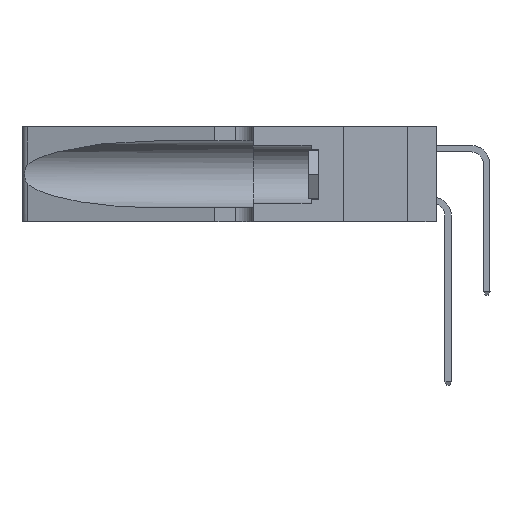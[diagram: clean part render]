
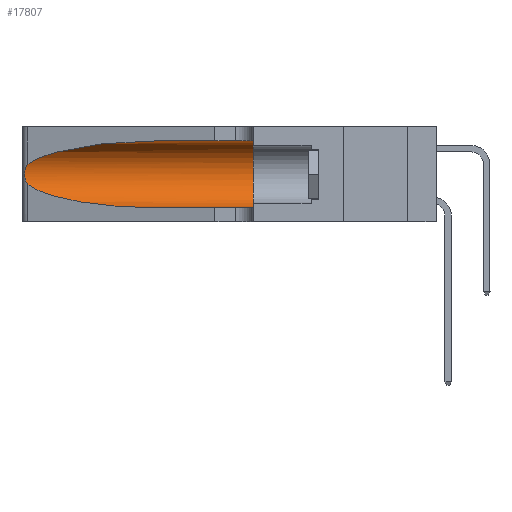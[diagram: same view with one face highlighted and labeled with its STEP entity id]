
A CAD part, left-side view. The second image highlights one B-rep face of the part: STEP entity #17807.
In plain terms, the highlighted cylindrical face has radius 3.308 mm (diameter 6.617 mm), a partial arc.
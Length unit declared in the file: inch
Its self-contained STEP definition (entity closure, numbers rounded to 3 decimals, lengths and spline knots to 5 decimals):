
#35 = CARTESIAN_POINT ( 'NONE',  ( 0.18966, 0.96281, 0.05475 ) ) ;
#333 = VERTEX_POINT ( 'NONE', #11581 ) ;
#340 = EDGE_CURVE ( 'NONE', #333, #13767, #14621, .T. ) ;
#461 = ORIENTED_EDGE ( 'NONE', *, *, #8582, .T. ) ;
#627 = CARTESIAN_POINT ( 'NONE',  ( 0.25487, 1.22718, 0.14631 ) ) ;
#986 = DIRECTION ( 'NONE',  ( 0., -1., 0. ) ) ;
#1318 = CARTESIAN_POINT ( 'NONE',  ( 0.25555, 1.22994, 0.2215 ) ) ;
#1397 = CARTESIAN_POINT ( 'NONE',  ( 0.25639, 1.23186, 0.15144 ) ) ;
#1609 =( BOUNDED_CURVE ( )  B_SPLINE_CURVE ( 3, ( #13322, #1792, #5315, #16548 ),
 .UNSPECIFIED., .F., .F. ) 
 B_SPLINE_CURVE_WITH_KNOTS ( ( 4, 4 ),
 ( 1.5708, 2.84003 ),
 .UNSPECIFIED. ) 
 CURVE ( )  GEOMETRIC_REPRESENTATION_ITEM ( )  RATIONAL_B_SPLINE_CURVE ( ( 1., 0.87, 0.87, 1. ) ) 
 REPRESENTATION_ITEM ( '' )  );
#1792 = CARTESIAN_POINT ( 'NONE',  ( 0.18966, 0.96281, 0.31525 ) ) ;
#2018 =( BOUNDED_CURVE ( )  B_SPLINE_CURVE ( 3, ( #6963, #11746, #35, #11812 ),
 .UNSPECIFIED., .F., .F. ) 
 B_SPLINE_CURVE_WITH_KNOTS ( ( 4, 4 ),
 ( 3.44316, 4.71239 ),
 .UNSPECIFIED. ) 
 CURVE ( )  GEOMETRIC_REPRESENTATION_ITEM ( )  RATIONAL_B_SPLINE_CURVE ( ( 1., 0.87, 0.87, 1. ) ) 
 REPRESENTATION_ITEM ( '' )  );
#3030 = B_SPLINE_CURVE_WITH_KNOTS ( 'NONE', 3,
 ( #12923, #1318, #4884, #16147, #6558, #17744, #8206, #19356, #9835, #20980, #11409, #1397, #12991, #3214 ),
 .UNSPECIFIED., .F., .F.,
 ( 4, 2, 2, 2, 2, 2, 4 ),
 ( 0., 0.00027, 0.00053, 0.00107, 0.0016, 0.00187, 0.00214 ),
 .UNSPECIFIED. ) ;
#3214 = CARTESIAN_POINT ( 'NONE',  ( 0.25487, 1.22718, 0.14631 ) ) ;
#3275 = DIRECTION ( 'NONE',  ( 0., -1., 0. ) ) ;
#3315 = VERTEX_POINT ( 'NONE', #16402 ) ;
#3650 = VERTEX_POINT ( 'NONE', #627 ) ;
#4501 = CARTESIAN_POINT ( 'NONE',  ( 0.1305, 1.61858, 0.185 ) ) ;
#4884 = CARTESIAN_POINT ( 'NONE',  ( 0.25639, 1.23184, 0.21858 ) ) ;
#5246 = ORIENTED_EDGE ( 'NONE', *, *, #14555, .T. ) ;
#5315 = CARTESIAN_POINT ( 'NONE',  ( 0.2373, 1.15595, 0.28018 ) ) ;
#6307 = CARTESIAN_POINT ( 'NONE',  ( 0.25487, 1.22718, 0.22369 ) ) ;
#6558 = CARTESIAN_POINT ( 'NONE',  ( 0.25854, 1.2359, 0.20912 ) ) ;
#6621 = CYLINDRICAL_SURFACE ( 'NONE', #16503, 0.13025 ) ;
#6963 = CARTESIAN_POINT ( 'NONE',  ( 0.25487, 1.22718, 0.14631 ) ) ;
#7875 = ORIENTED_EDGE ( 'NONE', *, *, #340, .F. ) ;
#8206 = CARTESIAN_POINT ( 'NONE',  ( 0.26075, 1.23896, 0.19203 ) ) ;
#8582 = EDGE_CURVE ( 'NONE', #20147, #3650, #3030, .T. ) ;
#9186 = EDGE_LOOP ( 'NONE', ( #5246, #461, #13705, #17351, #7875, #17955 ) ) ;
#9196 = VERTEX_POINT ( 'NONE', #9884 ) ;
#9835 = CARTESIAN_POINT ( 'NONE',  ( 0.26017, 1.23833, 0.17102 ) ) ;
#9884 = CARTESIAN_POINT ( 'NONE',  ( 0.1305, 0.72297, 0.05475 ) ) ;
#10000 = DIRECTION ( 'NONE',  ( 0., 0., 1. ) ) ;
#10018 = DIRECTION ( 'NONE',  ( 0., 1., 0. ) ) ;
#10058 = CARTESIAN_POINT ( 'NONE',  ( 0.1305, 0.35, 0.185 ) ) ;
#11079 = CARTESIAN_POINT ( 'NONE',  ( 0.1305, 0.35, 0.05475 ) ) ;
#11409 = CARTESIAN_POINT ( 'NONE',  ( 0.25789, 1.23486, 0.15765 ) ) ;
#11581 = CARTESIAN_POINT ( 'NONE',  ( 0.1305, 0.35, 0.31525 ) ) ;
#11746 = CARTESIAN_POINT ( 'NONE',  ( 0.2373, 1.15595, 0.08982 ) ) ;
#11812 = CARTESIAN_POINT ( 'NONE',  ( 0.1305, 0.72297, 0.05475 ) ) ;
#11880 = FACE_OUTER_BOUND ( 'NONE', #9186, .T. ) ;
#12124 = VECTOR ( 'NONE', #3275, 39.37008 ) ;
#12886 = EDGE_CURVE ( 'NONE', #3315, #333, #17711, .T. ) ;
#12923 = CARTESIAN_POINT ( 'NONE',  ( 0.25487, 1.22718, 0.22369 ) ) ;
#12957 = VECTOR ( 'NONE', #13812, 39.37008 ) ;
#12991 = CARTESIAN_POINT ( 'NONE',  ( 0.25555, 1.22993, 0.14849 ) ) ;
#13322 = CARTESIAN_POINT ( 'NONE',  ( 0.1305, 0.72297, 0.31525 ) ) ;
#13705 = ORIENTED_EDGE ( 'NONE', *, *, #14054, .T. ) ;
#13767 = VERTEX_POINT ( 'NONE', #11079 ) ;
#13812 = DIRECTION ( 'NONE',  ( 0., -1., 0. ) ) ;
#14054 = EDGE_CURVE ( 'NONE', #3650, #9196, #2018, .T. ) ;
#14445 = EDGE_CURVE ( 'NONE', #9196, #13767, #16877, .T. ) ;
#14555 = EDGE_CURVE ( 'NONE', #3315, #20147, #1609, .T. ) ;
#14621 = CIRCLE ( 'NONE', #19220, 0.13025 ) ;
#14667 = CARTESIAN_POINT ( 'NONE',  ( 0.1305, 1.61858, 0.05475 ) ) ;
#16147 = CARTESIAN_POINT ( 'NONE',  ( 0.25787, 1.23484, 0.2124 ) ) ;
#16402 = CARTESIAN_POINT ( 'NONE',  ( 0.1305, 0.72297, 0.31525 ) ) ;
#16503 = AXIS2_PLACEMENT_3D ( 'NONE', #4501, #986, #20576 ) ;
#16548 = CARTESIAN_POINT ( 'NONE',  ( 0.25487, 1.22718, 0.22369 ) ) ;
#16877 = LINE ( 'NONE', #14667, #12124 ) ;
#17031 = CARTESIAN_POINT ( 'NONE',  ( 0.1305, 1.61858, 0.31525 ) ) ;
#17351 = ORIENTED_EDGE ( 'NONE', *, *, #14445, .T. ) ;
#17711 = LINE ( 'NONE', #17031, #12957 ) ;
#17744 = CARTESIAN_POINT ( 'NONE',  ( 0.26018, 1.23835, 0.19895 ) ) ;
#17807 = ADVANCED_FACE ( 'NONE', ( #11880 ), #6621, .F. ) ;
#17955 = ORIENTED_EDGE ( 'NONE', *, *, #12886, .F. ) ;
#19220 = AXIS2_PLACEMENT_3D ( 'NONE', #10058, #10018, #10000 ) ;
#19356 = CARTESIAN_POINT ( 'NONE',  ( 0.26075, 1.23896, 0.178 ) ) ;
#20147 = VERTEX_POINT ( 'NONE', #6307 ) ;
#20576 = DIRECTION ( 'NONE',  ( 0., 0., -1. ) ) ;
#20980 = CARTESIAN_POINT ( 'NONE',  ( 0.25856, 1.23593, 0.16098 ) ) ;
